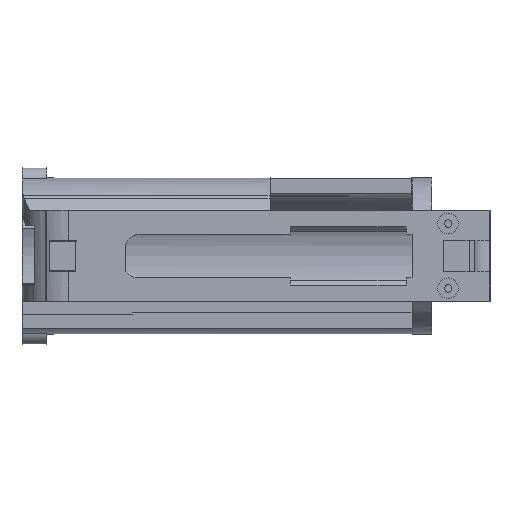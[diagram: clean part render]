
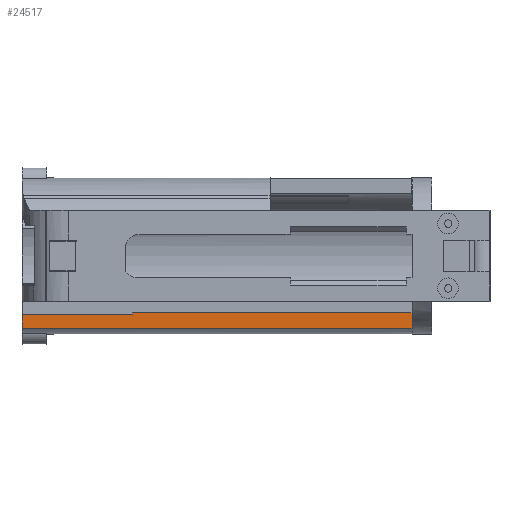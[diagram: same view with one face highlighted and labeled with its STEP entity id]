
A CAD part, front view. The second image highlights one B-rep face of the part: STEP entity #24517.
In plain terms, the highlighted planar face has unit normal (0, -1, 0).
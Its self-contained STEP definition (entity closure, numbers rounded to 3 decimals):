
#9340 = PLANE('',#9341);
#9341 = AXIS2_PLACEMENT_3D('',#9342,#9343,#9344);
#9342 = CARTESIAN_POINT('',(-19.05,12.674,-18.517));
#9343 = DIRECTION('',(1.,0.,0.));
#9344 = DIRECTION('',(0.,0.,1.));
#9909 = VERTEX_POINT('',#9910);
#9910 = CARTESIAN_POINT('',(-19.05,28.852,-29.496));
#9925 = CYLINDRICAL_SURFACE('',#9926,31.9);
#9926 = AXIS2_PLACEMENT_3D('',#9927,#9928,#9929);
#9927 = CARTESIAN_POINT('',(-19.05,41.,0.));
#9928 = DIRECTION('',(1.,0.,0.));
#9929 = DIRECTION('',(0.,-1.,0.));
#16067 = PLANE('',#16068);
#16068 = AXIS2_PLACEMENT_3D('',#16069,#16070,#16071);
#16069 = CARTESIAN_POINT('',(-177.75,19.308,23.389));
#16070 = DIRECTION('',(1.,0.,0.));
#16071 = DIRECTION('',(0.,0.,1.));
#17592 = EDGE_CURVE('',#17593,#9909,#17595,.T.);
#17593 = VERTEX_POINT('',#17594);
#17594 = CARTESIAN_POINT('',(-19.05,28.852,-23.101));
#17595 = SURFACE_CURVE('',#17596,(#17600,#17607),.PCURVE_S1.);
#17596 = LINE('',#17597,#17598);
#17597 = CARTESIAN_POINT('',(-19.05,28.852,-18.517));
#17598 = VECTOR('',#17599,1.);
#17599 = DIRECTION('',(0.,0.,-1.));
#17600 = PCURVE('',#9340,#17601);
#17601 = DEFINITIONAL_REPRESENTATION('',(#17602),#17606);
#17602 = LINE('',#17603,#17604);
#17603 = CARTESIAN_POINT('',(0.,-16.178));
#17604 = VECTOR('',#17605,1.);
#17605 = DIRECTION('',(-1.,0.));
#17606 = ( GEOMETRIC_REPRESENTATION_CONTEXT(2) 
PARAMETRIC_REPRESENTATION_CONTEXT() REPRESENTATION_CONTEXT('2D SPACE',''
  ) );
#17607 = PCURVE('',#17608,#17613);
#17608 = PLANE('',#17609);
#17609 = AXIS2_PLACEMENT_3D('',#17610,#17611,#17612);
#17610 = CARTESIAN_POINT('',(-177.75,28.852,-18.517));
#17611 = DIRECTION('',(0.,1.,0.));
#17612 = DIRECTION('',(0.,0.,-1.));
#17613 = DEFINITIONAL_REPRESENTATION('',(#17614),#17618);
#17614 = LINE('',#17615,#17616);
#17615 = CARTESIAN_POINT('',(0.,-158.7));
#17616 = VECTOR('',#17617,1.);
#17617 = DIRECTION('',(1.,0.));
#17618 = ( GEOMETRIC_REPRESENTATION_CONTEXT(2) 
PARAMETRIC_REPRESENTATION_CONTEXT() REPRESENTATION_CONTEXT('2D SPACE',''
  ) );
#17712 = VERTEX_POINT('',#17713);
#17713 = CARTESIAN_POINT('',(-177.75,28.852,-29.496));
#17739 = EDGE_CURVE('',#17712,#9909,#17740,.T.);
#17740 = SURFACE_CURVE('',#17741,(#17745,#17751),.PCURVE_S1.);
#17741 = LINE('',#17742,#17743);
#17742 = CARTESIAN_POINT('',(-19.05,28.852,-29.496));
#17743 = VECTOR('',#17744,1.);
#17744 = DIRECTION('',(1.,0.,0.));
#17745 = PCURVE('',#9925,#17746);
#17746 = DEFINITIONAL_REPRESENTATION('',(#17747),#17750);
#17747 = B_SPLINE_CURVE_WITH_KNOTS('',1,(#17748,#17749),.UNSPECIFIED.,
  .F.,.F.,(2,2),(-158.7,0.),
  .PIECEWISE_BEZIER_KNOTS.);
#17748 = CARTESIAN_POINT('',(-5.103,-158.7));
#17749 = CARTESIAN_POINT('',(-5.103,0.));
#17750 = ( GEOMETRIC_REPRESENTATION_CONTEXT(2) 
PARAMETRIC_REPRESENTATION_CONTEXT() REPRESENTATION_CONTEXT('2D SPACE',''
  ) );
#17751 = PCURVE('',#17608,#17752);
#17752 = DEFINITIONAL_REPRESENTATION('',(#17753),#17756);
#17753 = B_SPLINE_CURVE_WITH_KNOTS('',1,(#17754,#17755),.UNSPECIFIED.,
  .F.,.F.,(2,2),(-158.7,0.),
  .PIECEWISE_BEZIER_KNOTS.);
#17754 = CARTESIAN_POINT('',(10.979,0.));
#17755 = CARTESIAN_POINT('',(10.979,-158.7));
#17756 = ( GEOMETRIC_REPRESENTATION_CONTEXT(2) 
PARAMETRIC_REPRESENTATION_CONTEXT() REPRESENTATION_CONTEXT('2D SPACE',''
  ) );
#20602 = PLANE('',#20603);
#20603 = AXIS2_PLACEMENT_3D('',#20604,#20605,#20606);
#20604 = CARTESIAN_POINT('',(-177.75,28.852,-28.591));
#20605 = DIRECTION('',(0.,-1.,0.));
#20606 = DIRECTION('',(0.,0.,1.));
#21460 = VERTEX_POINT('',#21461);
#21461 = CARTESIAN_POINT('',(-177.75,28.852,-23.888));
#21498 = PLANE('',#21499);
#21499 = AXIS2_PLACEMENT_3D('',#21500,#21501,#21502);
#21500 = CARTESIAN_POINT('',(-177.75,19.308,23.389));
#21501 = DIRECTION('',(1.,0.,0.));
#21502 = DIRECTION('',(0.,0.,1.));
#23481 = VERTEX_POINT('',#23482);
#23482 = CARTESIAN_POINT('',(-177.75,28.852,-28.591));
#23503 = EDGE_CURVE('',#23481,#17712,#23504,.T.);
#23504 = SURFACE_CURVE('',#23505,(#23509,#23516),.PCURVE_S1.);
#23505 = LINE('',#23506,#23507);
#23506 = CARTESIAN_POINT('',(-177.75,28.852,-18.517));
#23507 = VECTOR('',#23508,1.);
#23508 = DIRECTION('',(0.,0.,-1.));
#23509 = PCURVE('',#16067,#23510);
#23510 = DEFINITIONAL_REPRESENTATION('',(#23511),#23515);
#23511 = LINE('',#23512,#23513);
#23512 = CARTESIAN_POINT('',(-41.906,-9.544));
#23513 = VECTOR('',#23514,1.);
#23514 = DIRECTION('',(-1.,0.));
#23515 = ( GEOMETRIC_REPRESENTATION_CONTEXT(2) 
PARAMETRIC_REPRESENTATION_CONTEXT() REPRESENTATION_CONTEXT('2D SPACE',''
  ) );
#23516 = PCURVE('',#17608,#23517);
#23517 = DEFINITIONAL_REPRESENTATION('',(#23518),#23522);
#23518 = LINE('',#23519,#23520);
#23519 = CARTESIAN_POINT('',(0.,0.));
#23520 = VECTOR('',#23521,1.);
#23521 = DIRECTION('',(1.,0.));
#23522 = ( GEOMETRIC_REPRESENTATION_CONTEXT(2) 
PARAMETRIC_REPRESENTATION_CONTEXT() REPRESENTATION_CONTEXT('2D SPACE',''
  ) );
#24517 = ADVANCED_FACE('',(#24518),#17608,.F.);
#24518 = FACE_BOUND('',#24519,.F.);
#24519 = EDGE_LOOP('',(#24520,#24541,#24563,#24585,#24605,#24606,#24607)
  );
#24520 = ORIENTED_EDGE('',*,*,#24521,.F.);
#24521 = EDGE_CURVE('',#21460,#23481,#24522,.T.);
#24522 = SURFACE_CURVE('',#24523,(#24527,#24534),.PCURVE_S1.);
#24523 = LINE('',#24524,#24525);
#24524 = CARTESIAN_POINT('',(-177.75,28.852,-18.517));
#24525 = VECTOR('',#24526,1.);
#24526 = DIRECTION('',(0.,0.,-1.));
#24527 = PCURVE('',#17608,#24528);
#24528 = DEFINITIONAL_REPRESENTATION('',(#24529),#24533);
#24529 = LINE('',#24530,#24531);
#24530 = CARTESIAN_POINT('',(0.,0.));
#24531 = VECTOR('',#24532,1.);
#24532 = DIRECTION('',(1.,0.));
#24533 = ( GEOMETRIC_REPRESENTATION_CONTEXT(2) 
PARAMETRIC_REPRESENTATION_CONTEXT() REPRESENTATION_CONTEXT('2D SPACE',''
  ) );
#24534 = PCURVE('',#21498,#24535);
#24535 = DEFINITIONAL_REPRESENTATION('',(#24536),#24540);
#24536 = LINE('',#24537,#24538);
#24537 = CARTESIAN_POINT('',(-41.906,-9.544));
#24538 = VECTOR('',#24539,1.);
#24539 = DIRECTION('',(-1.,0.));
#24540 = ( GEOMETRIC_REPRESENTATION_CONTEXT(2) 
PARAMETRIC_REPRESENTATION_CONTEXT() REPRESENTATION_CONTEXT('2D SPACE',''
  ) );
#24541 = ORIENTED_EDGE('',*,*,#24542,.T.);
#24542 = EDGE_CURVE('',#21460,#24543,#24545,.T.);
#24543 = VERTEX_POINT('',#24544);
#24544 = CARTESIAN_POINT('',(-132.75,28.852,-23.888));
#24545 = SURFACE_CURVE('',#24546,(#24550,#24557),.PCURVE_S1.);
#24546 = LINE('',#24547,#24548);
#24547 = CARTESIAN_POINT('',(-177.75,28.852,-23.888));
#24548 = VECTOR('',#24549,1.);
#24549 = DIRECTION('',(1.,0.,0.));
#24550 = PCURVE('',#17608,#24551);
#24551 = DEFINITIONAL_REPRESENTATION('',(#24552),#24556);
#24552 = LINE('',#24553,#24554);
#24553 = CARTESIAN_POINT('',(5.37,0.));
#24554 = VECTOR('',#24555,1.);
#24555 = DIRECTION('',(0.,-1.));
#24556 = ( GEOMETRIC_REPRESENTATION_CONTEXT(2) 
PARAMETRIC_REPRESENTATION_CONTEXT() REPRESENTATION_CONTEXT('2D SPACE',''
  ) );
#24557 = PCURVE('',#20602,#24558);
#24558 = DEFINITIONAL_REPRESENTATION('',(#24559),#24562);
#24559 = B_SPLINE_CURVE_WITH_KNOTS('',1,(#24560,#24561),.UNSPECIFIED.,
  .F.,.F.,(2,2),(-4.5,49.5),.PIECEWISE_BEZIER_KNOTS.);
#24560 = CARTESIAN_POINT('',(4.703,4.5));
#24561 = CARTESIAN_POINT('',(4.703,-49.5));
#24562 = ( GEOMETRIC_REPRESENTATION_CONTEXT(2) 
PARAMETRIC_REPRESENTATION_CONTEXT() REPRESENTATION_CONTEXT('2D SPACE',''
  ) );
#24563 = ORIENTED_EDGE('',*,*,#24564,.T.);
#24564 = EDGE_CURVE('',#24543,#24565,#24567,.T.);
#24565 = VERTEX_POINT('',#24566);
#24566 = CARTESIAN_POINT('',(-132.75,28.852,-23.101));
#24567 = SURFACE_CURVE('',#24568,(#24572,#24579),.PCURVE_S1.);
#24568 = LINE('',#24569,#24570);
#24569 = CARTESIAN_POINT('',(-132.75,28.852,-24.693));
#24570 = VECTOR('',#24571,1.);
#24571 = DIRECTION('',(0.,0.,1.));
#24572 = PCURVE('',#17608,#24573);
#24573 = DEFINITIONAL_REPRESENTATION('',(#24574),#24578);
#24574 = LINE('',#24575,#24576);
#24575 = CARTESIAN_POINT('',(6.176,-45.));
#24576 = VECTOR('',#24577,1.);
#24577 = DIRECTION('',(-1.,0.));
#24578 = ( GEOMETRIC_REPRESENTATION_CONTEXT(2) 
PARAMETRIC_REPRESENTATION_CONTEXT() REPRESENTATION_CONTEXT('2D SPACE',''
  ) );
#24579 = PCURVE('',#20602,#24580);
#24580 = DEFINITIONAL_REPRESENTATION('',(#24581),#24584);
#24581 = B_SPLINE_CURVE_WITH_KNOTS('',1,(#24582,#24583),.UNSPECIFIED.,
  .F.,.F.,(2,2),(-4.349,6.978),
  .PIECEWISE_BEZIER_KNOTS.);
#24582 = CARTESIAN_POINT('',(-0.451,-45.));
#24583 = CARTESIAN_POINT('',(10.876,-45.));
#24584 = ( GEOMETRIC_REPRESENTATION_CONTEXT(2) 
PARAMETRIC_REPRESENTATION_CONTEXT() REPRESENTATION_CONTEXT('2D SPACE',''
  ) );
#24585 = ORIENTED_EDGE('',*,*,#24586,.F.);
#24586 = EDGE_CURVE('',#17593,#24565,#24587,.T.);
#24587 = SURFACE_CURVE('',#24588,(#24592,#24599),.PCURVE_S1.);
#24588 = LINE('',#24589,#24590);
#24589 = CARTESIAN_POINT('',(-177.8,28.852,-23.101));
#24590 = VECTOR('',#24591,1.);
#24591 = DIRECTION('',(-1.,0.,0.));
#24592 = PCURVE('',#17608,#24593);
#24593 = DEFINITIONAL_REPRESENTATION('',(#24594),#24598);
#24594 = LINE('',#24595,#24596);
#24595 = CARTESIAN_POINT('',(4.583,0.05));
#24596 = VECTOR('',#24597,1.);
#24597 = DIRECTION('',(0.,1.));
#24598 = ( GEOMETRIC_REPRESENTATION_CONTEXT(2) 
PARAMETRIC_REPRESENTATION_CONTEXT() REPRESENTATION_CONTEXT('2D SPACE',''
  ) );
#24599 = PCURVE('',#20602,#24600);
#24600 = DEFINITIONAL_REPRESENTATION('',(#24601),#24604);
#24601 = B_SPLINE_CURVE_WITH_KNOTS('',1,(#24602,#24603),.UNSPECIFIED.,
  .F.,.F.,(2,2),(-158.755,0.),
  .PIECEWISE_BEZIER_KNOTS.);
#24602 = CARTESIAN_POINT('',(5.49,-158.705));
#24603 = CARTESIAN_POINT('',(5.49,0.05));
#24604 = ( GEOMETRIC_REPRESENTATION_CONTEXT(2) 
PARAMETRIC_REPRESENTATION_CONTEXT() REPRESENTATION_CONTEXT('2D SPACE',''
  ) );
#24605 = ORIENTED_EDGE('',*,*,#17592,.T.);
#24606 = ORIENTED_EDGE('',*,*,#17739,.F.);
#24607 = ORIENTED_EDGE('',*,*,#23503,.F.);
